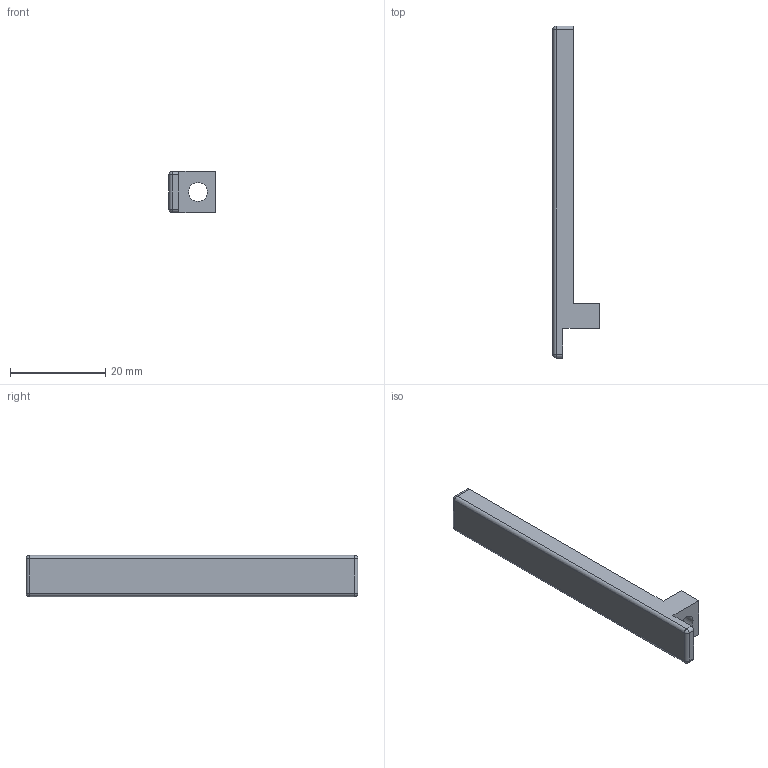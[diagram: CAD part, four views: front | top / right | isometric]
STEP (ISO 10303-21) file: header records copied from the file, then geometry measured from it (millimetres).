
FILE_DESCRIPTION (( 'STEP AP214' ), '1' );
FILE_NAME ('307-220-068.STEP', '2020-08-18T15:30:31', ( '' ), ( '' ), 'SwSTEP 2.0', 'SolidWorks 2020', '' );
FILE_SCHEMA (( 'AUTOMOTIVE_DESIGN' ));
Length unit declared in the file: inch
Products named in the file (1): 307-220-068
Bounding box: 9.75 x 69.85 x 8.71 mm (x, y, z)
Volume: 2399.9 mm3; surface area: 2203.9 mm2
Topology: 1 solids, 1 shells, 47 faces, 127 edges, 78 vertices
Faces by surface type: plane 28, cylinder 15, sphere 4
Entity records: 1475 total; most frequent: CARTESIAN_POINT 249, DIRECTION 249, ORIENTED_EDGE 246, EDGE_CURVE 123, LINE 93, VECTOR 93, VERTEX_POINT 78, AXIS2_PLACEMENT_3D 78
